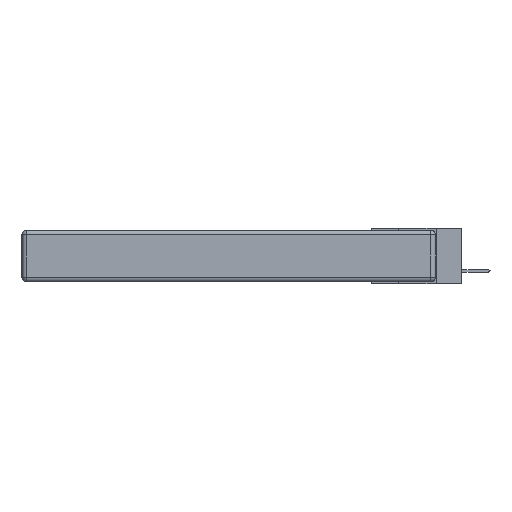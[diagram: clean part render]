
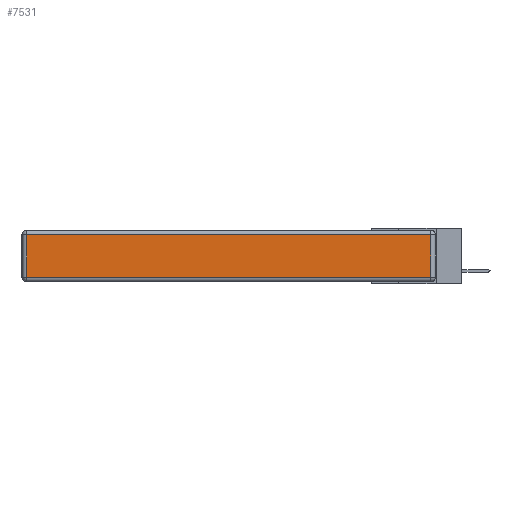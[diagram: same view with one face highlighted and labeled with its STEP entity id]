
A CAD part, left-side view. The second image highlights one B-rep face of the part: STEP entity #7531.
In plain terms, the highlighted planar face has unit normal (-1, 0, 0).
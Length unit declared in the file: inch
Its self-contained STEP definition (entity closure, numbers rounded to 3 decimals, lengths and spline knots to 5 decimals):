
#301 = CARTESIAN_POINT ( 'NONE',  ( 0., 0.03, -0.313 ) ) ;
#620 = CARTESIAN_POINT ( 'NONE',  ( 0., 2.75, -0.03 ) ) ;
#1090 = DIRECTION ( 'NONE',  ( 0., 0., 1. ) ) ;
#2007 = CARTESIAN_POINT ( 'NONE',  ( 0., 2.72, -0.343 ) ) ;
#2097 = DIRECTION ( 'NONE',  ( 0., 0., 1. ) ) ;
#3189 = VERTEX_POINT ( 'NONE', #24075 ) ;
#3997 = CARTESIAN_POINT ( 'NONE',  ( 0., 0.03, -0.343 ) ) ;
#4208 = LINE ( 'NONE', #24549, #9940 ) ;
#7257 = ORIENTED_EDGE ( 'NONE', *, *, #18077, .T. ) ;
#7473 = ORIENTED_EDGE ( 'NONE', *, *, #16744, .T. ) ;
#7531 = ADVANCED_FACE ( 'NONE', ( #17462 ), #23948, .T. ) ;
#7873 = EDGE_CURVE ( 'NONE', #3189, #17762, #4208, .T. ) ;
#8343 = LINE ( 'NONE', #2007, #20946 ) ;
#9933 = CARTESIAN_POINT ( 'NONE',  ( 0., 0.03, -0.03 ) ) ;
#9940 = VECTOR ( 'NONE', #26575, 39.37008 ) ;
#10616 = DIRECTION ( 'NONE',  ( 0., 1., 0. ) ) ;
#12791 = ORIENTED_EDGE ( 'NONE', *, *, #17296, .T. ) ;
#13344 = DIRECTION ( 'NONE',  ( -1., 0., 0. ) ) ;
#15766 = CARTESIAN_POINT ( 'NONE',  ( 0., 2.72, -0.03 ) ) ;
#16439 = DIRECTION ( 'NONE',  ( 0., 0., -1. ) ) ;
#16490 = ORIENTED_EDGE ( 'NONE', *, *, #7873, .T. ) ;
#16744 = EDGE_CURVE ( 'NONE', #19309, #3189, #8343, .T. ) ;
#17296 = EDGE_CURVE ( 'NONE', #26712, #19309, #21560, .T. ) ;
#17462 = FACE_OUTER_BOUND ( 'NONE', #18271, .T. ) ;
#17762 = VERTEX_POINT ( 'NONE', #301 ) ;
#18077 = EDGE_CURVE ( 'NONE', #17762, #26712, #24786, .T. ) ;
#18271 = EDGE_LOOP ( 'NONE', ( #16490, #7257, #12791, #7473 ) ) ;
#19279 = VECTOR ( 'NONE', #2097, 39.37008 ) ;
#19309 = VERTEX_POINT ( 'NONE', #15766 ) ;
#20946 = VECTOR ( 'NONE', #16439, 39.37008 ) ;
#21560 = LINE ( 'NONE', #620, #25169 ) ;
#22607 = AXIS2_PLACEMENT_3D ( 'NONE', #25982, #13344, #1090 ) ;
#23948 = PLANE ( 'NONE',  #22607 ) ;
#24075 = CARTESIAN_POINT ( 'NONE',  ( 0., 2.72, -0.313 ) ) ;
#24549 = CARTESIAN_POINT ( 'NONE',  ( 0., 0., -0.313 ) ) ;
#24786 = LINE ( 'NONE', #3997, #19279 ) ;
#25169 = VECTOR ( 'NONE', #10616, 39.37008 ) ;
#25982 = CARTESIAN_POINT ( 'NONE',  ( 0., 0., -0.343 ) ) ;
#26575 = DIRECTION ( 'NONE',  ( 0., -1., 0. ) ) ;
#26712 = VERTEX_POINT ( 'NONE', #9933 ) ;
